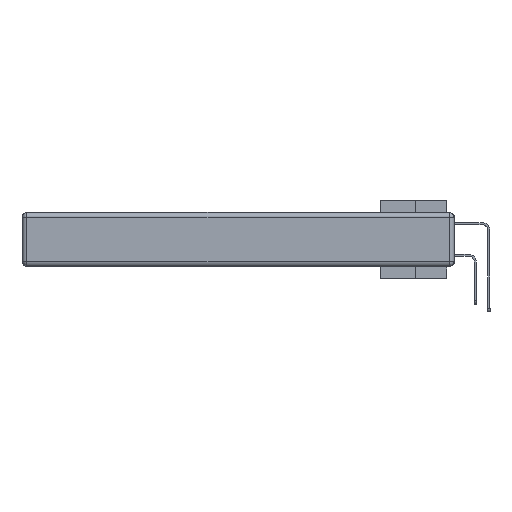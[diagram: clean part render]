
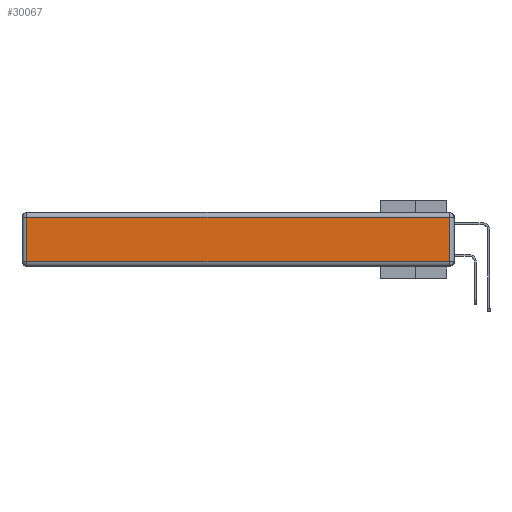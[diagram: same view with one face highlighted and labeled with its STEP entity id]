
A CAD part, left-side view. The second image highlights one B-rep face of the part: STEP entity #30067.
In plain terms, the highlighted planar face has unit normal (-1, 0, 0).
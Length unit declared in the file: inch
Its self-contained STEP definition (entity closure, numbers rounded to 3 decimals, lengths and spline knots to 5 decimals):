
#1058 = EDGE_CURVE ( 'NONE', #31709, #22051, #10973, .T. ) ;
#1336 = DIRECTION ( 'NONE',  ( 0., 0., 1. ) ) ;
#2116 = CARTESIAN_POINT ( 'NONE',  ( 0., 2.72, -0.03 ) ) ;
#6199 = LINE ( 'NONE', #16669, #17459 ) ;
#8561 = CARTESIAN_POINT ( 'NONE',  ( 0., 2.75, -0.03 ) ) ;
#8736 = EDGE_CURVE ( 'NONE', #22051, #33823, #6199, .T. ) ;
#8956 = DIRECTION ( 'NONE',  ( 0., 0., -1. ) ) ;
#9294 = CARTESIAN_POINT ( 'NONE',  ( 0., 0., -0.343 ) ) ;
#9301 = CARTESIAN_POINT ( 'NONE',  ( 0., 0.03, -0.343 ) ) ;
#10973 = LINE ( 'NONE', #8561, #22017 ) ;
#11971 = LINE ( 'NONE', #30440, #23292 ) ;
#12137 = DIRECTION ( 'NONE',  ( 0., -1., 0. ) ) ;
#12275 = ORIENTED_EDGE ( 'NONE', *, *, #1058, .T. ) ;
#13462 = EDGE_CURVE ( 'NONE', #33823, #15017, #11971, .T. ) ;
#13631 = ORIENTED_EDGE ( 'NONE', *, *, #8736, .T. ) ;
#13885 = DIRECTION ( 'NONE',  ( 0., 1., 0. ) ) ;
#14416 = VECTOR ( 'NONE', #27623, 39.37008 ) ;
#15017 = VERTEX_POINT ( 'NONE', #17066 ) ;
#16669 = CARTESIAN_POINT ( 'NONE',  ( 0., 2.72, -0.343 ) ) ;
#17066 = CARTESIAN_POINT ( 'NONE',  ( 0., 0.03, -0.313 ) ) ;
#17459 = VECTOR ( 'NONE', #8956, 39.37008 ) ;
#19243 = FACE_OUTER_BOUND ( 'NONE', #30173, .T. ) ;
#20461 = CARTESIAN_POINT ( 'NONE',  ( 0., 0.03, -0.03 ) ) ;
#22017 = VECTOR ( 'NONE', #13885, 39.37008 ) ;
#22051 = VERTEX_POINT ( 'NONE', #2116 ) ;
#22487 = LINE ( 'NONE', #9301, #14416 ) ;
#22902 = EDGE_CURVE ( 'NONE', #15017, #31709, #22487, .T. ) ;
#23292 = VECTOR ( 'NONE', #12137, 39.37008 ) ;
#27623 = DIRECTION ( 'NONE',  ( 0., 0., 1. ) ) ;
#28525 = ORIENTED_EDGE ( 'NONE', *, *, #13462, .T. ) ;
#29207 = ORIENTED_EDGE ( 'NONE', *, *, #22902, .T. ) ;
#29839 = CARTESIAN_POINT ( 'NONE',  ( 0., 2.72, -0.313 ) ) ;
#30067 = ADVANCED_FACE ( 'NONE', ( #19243 ), #32421, .T. ) ;
#30173 = EDGE_LOOP ( 'NONE', ( #28525, #29207, #12275, #13631 ) ) ;
#30440 = CARTESIAN_POINT ( 'NONE',  ( 0., 0., -0.313 ) ) ;
#31709 = VERTEX_POINT ( 'NONE', #20461 ) ;
#32275 = AXIS2_PLACEMENT_3D ( 'NONE', #9294, #32755, #1336 ) ;
#32421 = PLANE ( 'NONE',  #32275 ) ;
#32755 = DIRECTION ( 'NONE',  ( -1., 0., 0. ) ) ;
#33823 = VERTEX_POINT ( 'NONE', #29839 ) ;
